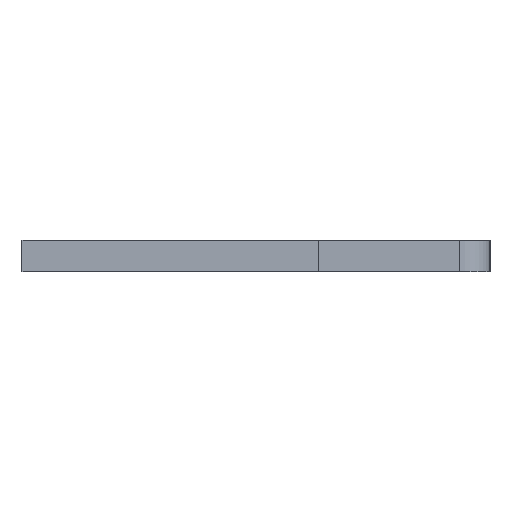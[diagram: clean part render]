
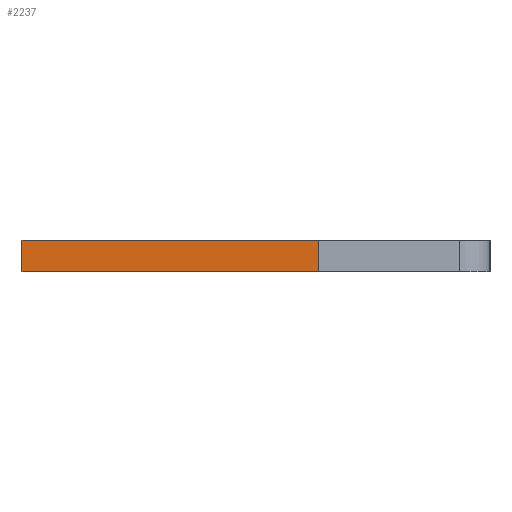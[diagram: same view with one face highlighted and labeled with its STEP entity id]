
A CAD part, left-side view. The second image highlights one B-rep face of the part: STEP entity #2237.
In plain terms, the highlighted face is planar.
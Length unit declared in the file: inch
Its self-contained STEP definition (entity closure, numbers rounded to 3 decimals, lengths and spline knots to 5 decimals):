
#72 = ORIENTED_EDGE ( 'NONE', *, *, #2603, .T. ) ;
#104 = ORIENTED_EDGE ( 'NONE', *, *, #390, .T. ) ;
#242 = CARTESIAN_POINT ( 'NONE',  ( 0.01, 0.15, -0.04 ) ) ;
#263 = DIRECTION ( 'NONE',  ( 0., 0., 1. ) ) ;
#264 = EDGE_CURVE ( 'NONE', #396, #1831, #1363, .T. ) ;
#373 = VECTOR ( 'NONE', #500, 39.37008 ) ;
#390 = EDGE_CURVE ( 'NONE', #2553, #810, #2585, .T. ) ;
#396 = VERTEX_POINT ( 'NONE', #2465 ) ;
#436 = CARTESIAN_POINT ( 'NONE',  ( 0.01, 0.15, -0.04 ) ) ;
#447 = DIRECTION ( 'NONE',  ( -1., 0., 0. ) ) ;
#500 = DIRECTION ( 'NONE',  ( -1., 0., 0. ) ) ;
#519 = DIRECTION ( 'NONE',  ( 0., 1., 0. ) ) ;
#685 = CARTESIAN_POINT ( 'NONE',  ( -0.01, -0.04, -0.04 ) ) ;
#710 = VECTOR ( 'NONE', #2187, 39.37008 ) ;
#759 = FACE_OUTER_BOUND ( 'NONE', #876, .T. ) ;
#810 = VERTEX_POINT ( 'NONE', #2576 ) ;
#848 = LINE ( 'NONE', #2364, #373 ) ;
#873 = AXIS2_PLACEMENT_3D ( 'NONE', #1501, #263, #1126 ) ;
#876 = EDGE_LOOP ( 'NONE', ( #104, #1230, #2195, #72 ) ) ;
#1126 = DIRECTION ( 'NONE',  ( 1., 0., 0. ) ) ;
#1146 = CARTESIAN_POINT ( 'NONE',  ( 0.01, 0.15, -0.04 ) ) ;
#1230 = ORIENTED_EDGE ( 'NONE', *, *, #2121, .F. ) ;
#1315 = PLANE ( 'NONE',  #873 ) ;
#1363 = LINE ( 'NONE', #1146, #1857 ) ;
#1501 = CARTESIAN_POINT ( 'NONE',  ( 0.01, 0.15, -0.04 ) ) ;
#1529 = CARTESIAN_POINT ( 'NONE',  ( -0.01, 0.15, -0.04 ) ) ;
#1831 = VERTEX_POINT ( 'NONE', #436 ) ;
#1857 = VECTOR ( 'NONE', #519, 39.37008 ) ;
#1999 = LINE ( 'NONE', #242, #2358 ) ;
#2121 = EDGE_CURVE ( 'NONE', #1831, #810, #1999, .T. ) ;
#2187 = DIRECTION ( 'NONE',  ( 0., 1., 0. ) ) ;
#2195 = ORIENTED_EDGE ( 'NONE', *, *, #264, .F. ) ;
#2237 = ADVANCED_FACE ( 'NONE', ( #759 ), #1315, .F. ) ;
#2358 = VECTOR ( 'NONE', #447, 39.37008 ) ;
#2364 = CARTESIAN_POINT ( 'NONE',  ( 0.01, -0.04, -0.04 ) ) ;
#2465 = CARTESIAN_POINT ( 'NONE',  ( 0.01, -0.04, -0.04 ) ) ;
#2553 = VERTEX_POINT ( 'NONE', #685 ) ;
#2576 = CARTESIAN_POINT ( 'NONE',  ( -0.01, 0.15, -0.04 ) ) ;
#2585 = LINE ( 'NONE', #1529, #710 ) ;
#2603 = EDGE_CURVE ( 'NONE', #396, #2553, #848, .T. ) ;
